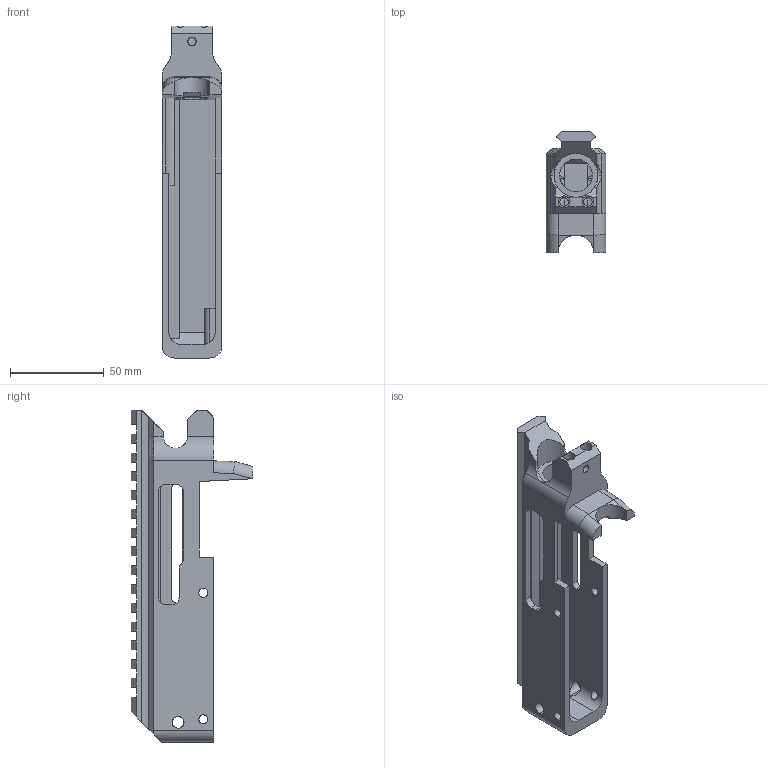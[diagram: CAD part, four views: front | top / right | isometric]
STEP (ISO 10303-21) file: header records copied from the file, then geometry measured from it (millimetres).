
FILE_DESCRIPTION(/* description */ ('Alibre Inc.'),/* implementation_level */ '2;1');
FILE_NAME(/* name */ 'export0',/* time_stamp */ '2012-04-27T10:01:53-05:00',/* author */ (''),/* organization */ (''),/* preprocessor_version */ 'ST-DEVELOPER v14',/* originating_system */ 'Alibre',/* authorisation */ '');
FILE_SCHEMA (('AUTOMOTIVE_DESIGN'));
Length unit declared in the file: inch
Bounding box: 31.75 x 64.9 x 176.91 mm (x, y, z)
Volume: 93071.3 mm3; surface area: 40160.1 mm2
Topology: 1 solids, 1 shells, 241 faces, 707 edges, 458 vertices
Faces by surface type: plane 170, cylinder 63, cone 8
Entity records: 8114 total; most frequent: CARTESIAN_POINT 1882, ORIENTED_EDGE 1406, DIRECTION 1075, EDGE_CURVE 703, VECTOR 542, LINE 542, VERTEX_POINT 458, AXIS2_PLACEMENT_3D 350
